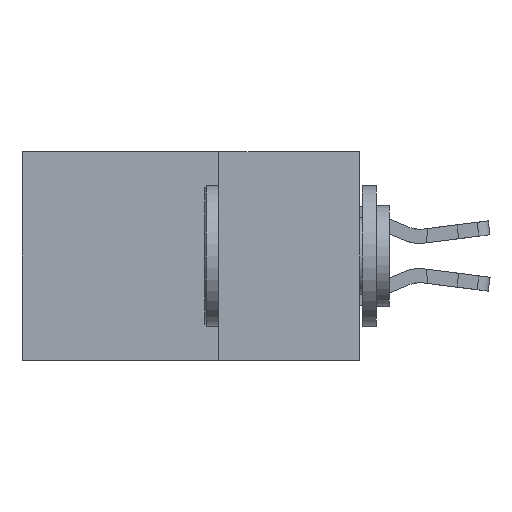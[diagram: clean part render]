
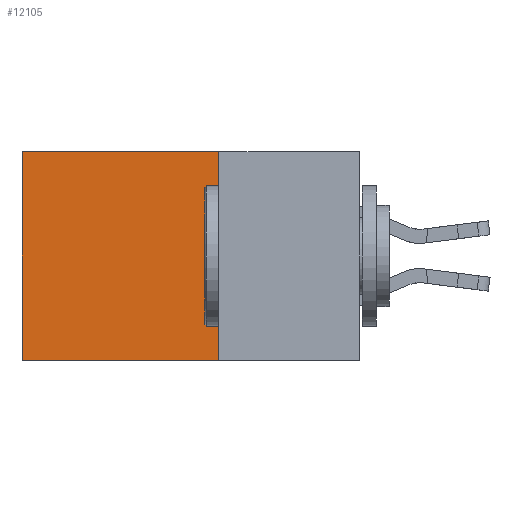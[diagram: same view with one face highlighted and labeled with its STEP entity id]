
A CAD part, left-side view. The second image highlights one B-rep face of the part: STEP entity #12105.
In plain terms, the highlighted planar face has unit normal (-1, 0, 0).
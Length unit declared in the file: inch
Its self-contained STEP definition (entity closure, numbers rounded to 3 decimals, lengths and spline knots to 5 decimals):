
#118 = CARTESIAN_POINT ( 'NONE',  ( 0.2875, 0.25, -0.37 ) ) ;
#576 = PLANE ( 'NONE',  #13655 ) ;
#1475 = VECTOR ( 'NONE', #2152, 39.37008 ) ;
#1926 = CARTESIAN_POINT ( 'NONE',  ( 0.2875, 0.25, 0. ) ) ;
#2152 = DIRECTION ( 'NONE',  ( 0., 1., 0. ) ) ;
#2912 = CARTESIAN_POINT ( 'NONE',  ( 0.2875, 0.25, 0. ) ) ;
#3011 = VERTEX_POINT ( 'NONE', #19315 ) ;
#4348 = DIRECTION ( 'NONE',  ( 0., 0., -1. ) ) ;
#4416 = EDGE_LOOP ( 'NONE', ( #13967, #11618, #15444, #8662 ) ) ;
#4669 = DIRECTION ( 'NONE',  ( 1., 0., 0. ) ) ;
#4929 = CARTESIAN_POINT ( 'NONE',  ( 0.2875, 0.25, 0. ) ) ;
#5913 = LINE ( 'NONE', #4929, #16121 ) ;
#6586 = LINE ( 'NONE', #118, #1475 ) ;
#7912 = EDGE_CURVE ( 'NONE', #22078, #7972, #6586, .T. ) ;
#7972 = VERTEX_POINT ( 'NONE', #15739 ) ;
#8537 = VERTEX_POINT ( 'NONE', #2912 ) ;
#8662 = ORIENTED_EDGE ( 'NONE', *, *, #12218, .T. ) ;
#10125 = DIRECTION ( 'NONE',  ( 0., 0., -1. ) ) ;
#11345 = FACE_OUTER_BOUND ( 'NONE', #4416, .T. ) ;
#11618 = ORIENTED_EDGE ( 'NONE', *, *, #7912, .F. ) ;
#12105 = ADVANCED_FACE ( 'NONE', ( #11345 ), #576, .F. ) ;
#12218 = EDGE_CURVE ( 'NONE', #8537, #3011, #14032, .T. ) ;
#13655 = AXIS2_PLACEMENT_3D ( 'NONE', #23751, #4669, #4348 ) ;
#13967 = ORIENTED_EDGE ( 'NONE', *, *, #18794, .T. ) ;
#14032 = LINE ( 'NONE', #1926, #20373 ) ;
#15444 = ORIENTED_EDGE ( 'NONE', *, *, #24501, .F. ) ;
#15739 = CARTESIAN_POINT ( 'NONE',  ( 0.2875, 0.6, -0.37 ) ) ;
#16121 = VECTOR ( 'NONE', #18362, 39.37008 ) ;
#17212 = DIRECTION ( 'NONE',  ( 0., 1., 0. ) ) ;
#17739 = CARTESIAN_POINT ( 'NONE',  ( 0.2875, 0.25, -0.37 ) ) ;
#17898 = CARTESIAN_POINT ( 'NONE',  ( 0.2875, 0.6, 0. ) ) ;
#18189 = VECTOR ( 'NONE', #10125, 39.37008 ) ;
#18362 = DIRECTION ( 'NONE',  ( 0., 0., -1. ) ) ;
#18794 = EDGE_CURVE ( 'NONE', #3011, #7972, #22363, .T. ) ;
#19315 = CARTESIAN_POINT ( 'NONE',  ( 0.2875, 0.6, 0. ) ) ;
#20373 = VECTOR ( 'NONE', #17212, 39.37008 ) ;
#22078 = VERTEX_POINT ( 'NONE', #17739 ) ;
#22363 = LINE ( 'NONE', #17898, #18189 ) ;
#23751 = CARTESIAN_POINT ( 'NONE',  ( 0.2875, 0.25, 0. ) ) ;
#24501 = EDGE_CURVE ( 'NONE', #8537, #22078, #5913, .T. ) ;
